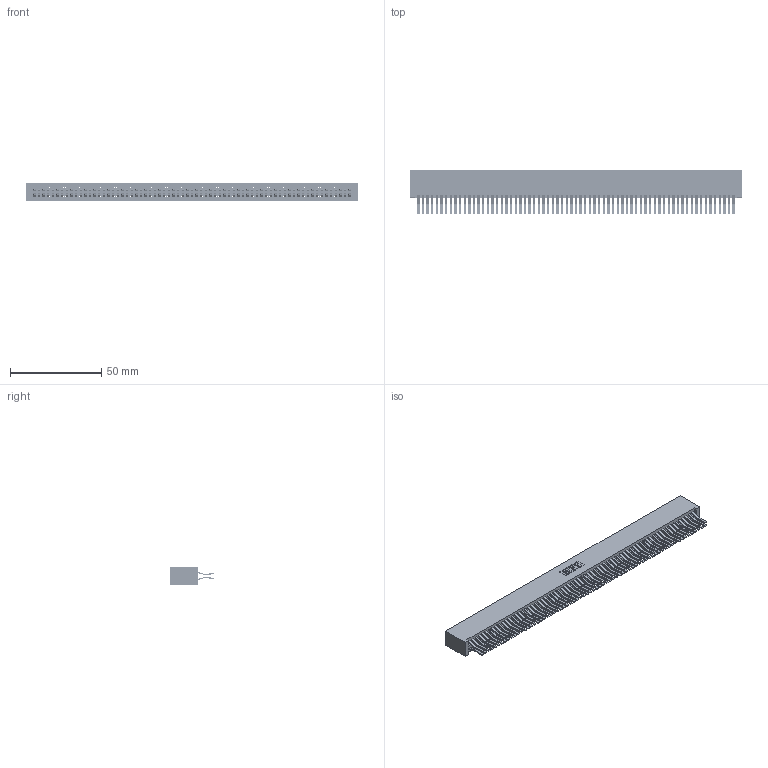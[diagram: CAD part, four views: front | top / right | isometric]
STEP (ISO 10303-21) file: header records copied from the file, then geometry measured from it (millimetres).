
FILE_DESCRIPTION (( 'STEP AP203' ), '1' );
FILE_NAME ('395-138-560-201.STEP', '2018-12-05T18:31:01', ( '' ), ( '' ), 'SwSTEP 2.0', 'SolidWorks 2016', '' );
FILE_SCHEMA (( 'CONFIG_CONTROL_DESIGN' ));
Length unit declared in the file: inch
Products named in the file (3): 395-138-560-201; 345 Part_No Mounting Lugs; 345-292-001_560 Tail
Assembly tree (139 placements, depth 2):
  395-138-560-201
    345 Part_No Mounting Lugs
    345-292-001_560 Tail  x138
Bounding box: 181.86 x 24.45 x 9.4 mm (x, y, z)
Volume: 19437.5 mm3; surface area: 31884.5 mm2
Topology: 139 solids, 139 shells, 7294 faces, 21707 edges, 14286 vertices
Faces by surface type: plane 4630, cylinder 2664
Entity records: 50315 total; most frequent: CARTESIAN_POINT 8408, ORIENTED_EDGE 8342, DIRECTION 7379, EDGE_CURVE 4171, LINE 3767, VECTOR 3767, VERTEX_POINT 2778, AXIS2_PLACEMENT_3D 1806
